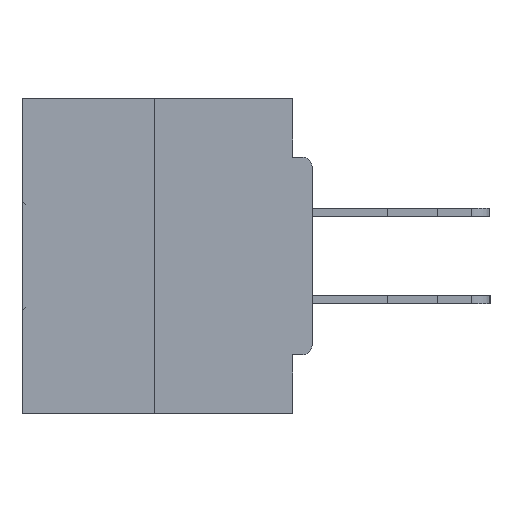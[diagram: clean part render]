
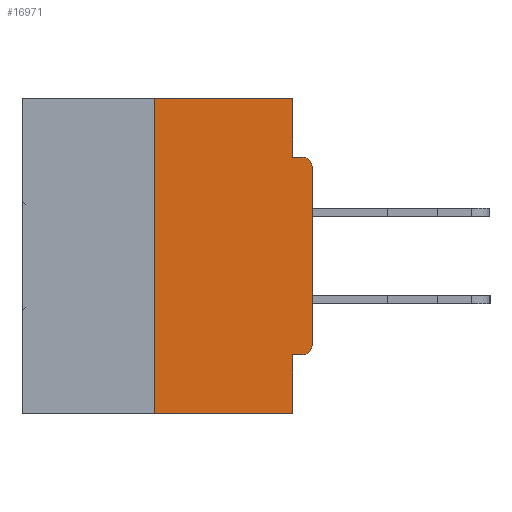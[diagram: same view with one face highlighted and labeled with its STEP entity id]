
A CAD part, left-side view. The second image highlights one B-rep face of the part: STEP entity #16971.
In plain terms, the highlighted planar face has unit normal (-1, 0, 0).
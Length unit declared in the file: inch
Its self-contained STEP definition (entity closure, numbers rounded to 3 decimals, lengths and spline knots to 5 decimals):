
#247 = EDGE_CURVE ( 'NONE', #21105, #28392, #38366, .T. ) ;
#647 = CARTESIAN_POINT ( 'NONE',  ( 0., 0.031, -0.5 ) ) ;
#953 = AXIS2_PLACEMENT_3D ( 'NONE', #20241, #14012, #10216 ) ;
#2009 = EDGE_CURVE ( 'NONE', #6304, #11280, #42902, .T. ) ;
#2400 = ORIENTED_EDGE ( 'NONE', *, *, #17751, .F. ) ;
#3037 = DIRECTION ( 'NONE',  ( 0., 0., -1. ) ) ;
#3525 = EDGE_CURVE ( 'NONE', #13699, #38555, #36416, .T. ) ;
#6131 = ORIENTED_EDGE ( 'NONE', *, *, #6601, .T. ) ;
#6304 = VERTEX_POINT ( 'NONE', #29802 ) ;
#6374 = DIRECTION ( 'NONE',  ( 0., 0., 1. ) ) ;
#6601 = EDGE_CURVE ( 'NONE', #8939, #11280, #35052, .T. ) ;
#7148 = ORIENTED_EDGE ( 'NONE', *, *, #247, .T. ) ;
#7286 = CIRCLE ( 'NONE', #20110, 0.015 ) ;
#7520 = CARTESIAN_POINT ( 'NONE',  ( 0., 0., -0.1085 ) ) ;
#7855 = CARTESIAN_POINT ( 'NONE',  ( 0., 0., 0. ) ) ;
#8412 = AXIS2_PLACEMENT_3D ( 'NONE', #42394, #35670, #22586 ) ;
#8608 = DIRECTION ( 'NONE',  ( 0., 0., -1. ) ) ;
#8703 = DIRECTION ( 'NONE',  ( 0., 0., -1. ) ) ;
#8939 = VERTEX_POINT ( 'NONE', #29206 ) ;
#9022 = VECTOR ( 'NONE', #6374, 39.37008 ) ;
#9697 = EDGE_CURVE ( 'NONE', #10341, #13699, #35123, .T. ) ;
#9839 = ORIENTED_EDGE ( 'NONE', *, *, #2009, .F. ) ;
#9869 = CARTESIAN_POINT ( 'NONE',  ( 0., 0.031, -0.0935 ) ) ;
#10177 = CARTESIAN_POINT ( 'NONE',  ( 0., 0.25, 0. ) ) ;
#10216 = DIRECTION ( 'NONE',  ( 0., 0., -1. ) ) ;
#10341 = VERTEX_POINT ( 'NONE', #31670 ) ;
#10736 = VECTOR ( 'NONE', #41145, 39.37008 ) ;
#11280 = VERTEX_POINT ( 'NONE', #647 ) ;
#11447 = CARTESIAN_POINT ( 'NONE',  ( 0., 0.015, -0.0935 ) ) ;
#11501 = CARTESIAN_POINT ( 'NONE',  ( 0., 0.031, -0.5 ) ) ;
#11954 = CARTESIAN_POINT ( 'NONE',  ( 0., 0.031, 0. ) ) ;
#13087 = VECTOR ( 'NONE', #23919, 39.37008 ) ;
#13676 = DIRECTION ( 'NONE',  ( 0., 0., 1. ) ) ;
#13699 = VERTEX_POINT ( 'NONE', #11954 ) ;
#14012 = DIRECTION ( 'NONE',  ( 1., 0., 0. ) ) ;
#15678 = CARTESIAN_POINT ( 'NONE',  ( 0., 0.46, -0.5 ) ) ;
#16720 = ORIENTED_EDGE ( 'NONE', *, *, #23398, .F. ) ;
#16971 = ADVANCED_FACE ( 'NONE', ( #17558 ), #23570, .F. ) ;
#17558 = FACE_OUTER_BOUND ( 'NONE', #36235, .T. ) ;
#17751 = EDGE_CURVE ( 'NONE', #38555, #21551, #40402, .T. ) ;
#19953 = CARTESIAN_POINT ( 'NONE',  ( 0., 0., -0.4065 ) ) ;
#20110 = AXIS2_PLACEMENT_3D ( 'NONE', #39185, #36076, #8703 ) ;
#20241 = CARTESIAN_POINT ( 'NONE',  ( 0., 0.46, 0. ) ) ;
#20253 = CARTESIAN_POINT ( 'NONE',  ( 0., 0.015, -0.4065 ) ) ;
#21105 = VERTEX_POINT ( 'NONE', #24002 ) ;
#21151 = VECTOR ( 'NONE', #40000, 39.37008 ) ;
#21551 = VERTEX_POINT ( 'NONE', #11447 ) ;
#22159 = ORIENTED_EDGE ( 'NONE', *, *, #24166, .F. ) ;
#22586 = DIRECTION ( 'NONE',  ( 0., 0., -1. ) ) ;
#22870 = LINE ( 'NONE', #10177, #9022 ) ;
#23398 = EDGE_CURVE ( 'NONE', #8939, #10341, #22870, .T. ) ;
#23570 = PLANE ( 'NONE',  #953 ) ;
#23919 = DIRECTION ( 'NONE',  ( 0., -1., 0. ) ) ;
#24002 = CARTESIAN_POINT ( 'NONE',  ( 0., 0., -0.3915 ) ) ;
#24166 = EDGE_CURVE ( 'NONE', #25150, #6304, #32859, .T. ) ;
#25150 = VERTEX_POINT ( 'NONE', #20253 ) ;
#26590 = VECTOR ( 'NONE', #8608, 39.37008 ) ;
#27606 = CIRCLE ( 'NONE', #8412, 0.015 ) ;
#27853 = VECTOR ( 'NONE', #13676, 39.37008 ) ;
#28392 = VERTEX_POINT ( 'NONE', #7520 ) ;
#28435 = CARTESIAN_POINT ( 'NONE',  ( 0., 0.46, 0. ) ) ;
#29206 = CARTESIAN_POINT ( 'NONE',  ( 0., 0.25, -0.5 ) ) ;
#29802 = CARTESIAN_POINT ( 'NONE',  ( 0., 0.031, -0.4065 ) ) ;
#31175 = ORIENTED_EDGE ( 'NONE', *, *, #3525, .F. ) ;
#31670 = CARTESIAN_POINT ( 'NONE',  ( 0., 0.25, 0. ) ) ;
#31777 = DIRECTION ( 'NONE',  ( 0., -1., 0. ) ) ;
#32508 = ORIENTED_EDGE ( 'NONE', *, *, #37113, .T. ) ;
#32859 = LINE ( 'NONE', #19953, #21151 ) ;
#33747 = CARTESIAN_POINT ( 'NONE',  ( 0., 0.031, 0. ) ) ;
#34497 = VECTOR ( 'NONE', #31777, 39.37008 ) ;
#34544 = ORIENTED_EDGE ( 'NONE', *, *, #9697, .F. ) ;
#35052 = LINE ( 'NONE', #15678, #10736 ) ;
#35123 = LINE ( 'NONE', #28435, #34497 ) ;
#35670 = DIRECTION ( 'NONE',  ( -1., 0., 0. ) ) ;
#36076 = DIRECTION ( 'NONE',  ( -1., 0., 0. ) ) ;
#36235 = EDGE_LOOP ( 'NONE', ( #34544, #16720, #6131, #9839, #22159, #43001, #7148, #32508, #2400, #31175 ) ) ;
#36416 = LINE ( 'NONE', #33747, #39348 ) ;
#36828 = CARTESIAN_POINT ( 'NONE',  ( 0., 0., -0.0935 ) ) ;
#37113 = EDGE_CURVE ( 'NONE', #28392, #21551, #27606, .T. ) ;
#38366 = LINE ( 'NONE', #7855, #27853 ) ;
#38555 = VERTEX_POINT ( 'NONE', #9869 ) ;
#39185 = CARTESIAN_POINT ( 'NONE',  ( 0., 0.015, -0.3915 ) ) ;
#39348 = VECTOR ( 'NONE', #3037, 39.37008 ) ;
#40000 = DIRECTION ( 'NONE',  ( 0., 1., 0. ) ) ;
#40402 = LINE ( 'NONE', #36828, #13087 ) ;
#41145 = DIRECTION ( 'NONE',  ( 0., -1., 0. ) ) ;
#41584 = EDGE_CURVE ( 'NONE', #25150, #21105, #7286, .T. ) ;
#42394 = CARTESIAN_POINT ( 'NONE',  ( 0., 0.015, -0.1085 ) ) ;
#42902 = LINE ( 'NONE', #11501, #26590 ) ;
#43001 = ORIENTED_EDGE ( 'NONE', *, *, #41584, .T. ) ;
